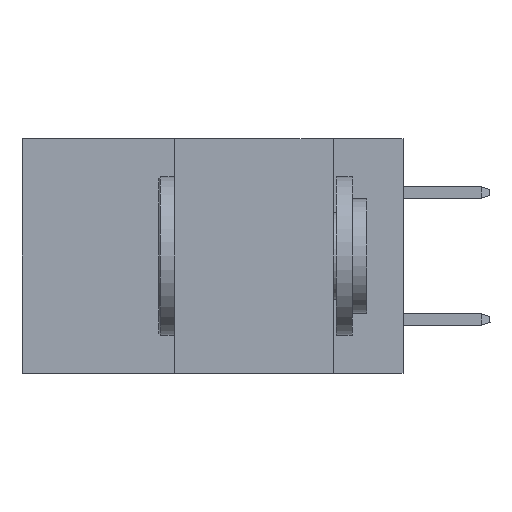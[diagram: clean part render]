
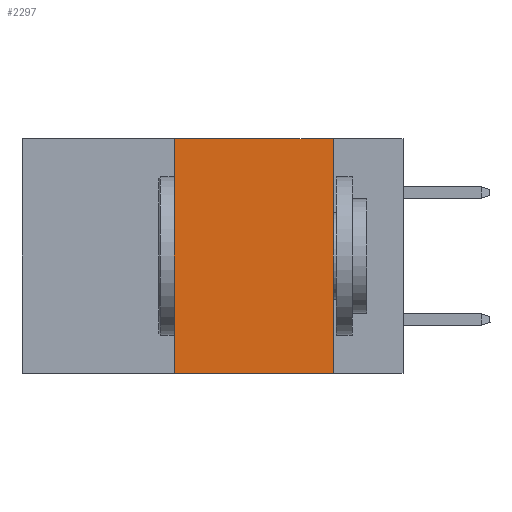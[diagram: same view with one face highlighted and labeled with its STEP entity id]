
A CAD part, left-side view. The second image highlights one B-rep face of the part: STEP entity #2297.
In plain terms, the highlighted planar face has unit normal (-1, 0, 0).
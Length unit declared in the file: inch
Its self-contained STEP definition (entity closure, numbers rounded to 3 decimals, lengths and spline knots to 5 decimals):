
#376 = VECTOR ( 'NONE', #2473, 39.37008 ) ;
#1329 = VECTOR ( 'NONE', #12461, 39.37008 ) ;
#2227 = EDGE_CURVE ( 'NONE', #12888, #9036, #9628, .T. ) ;
#2297 = ADVANCED_FACE ( 'NONE', ( #7451 ), #6273, .F. ) ;
#2473 = DIRECTION ( 'NONE',  ( 0., 0., -1. ) ) ;
#2727 = AXIS2_PLACEMENT_3D ( 'NONE', #7508, #8584, #14668 ) ;
#3053 = CARTESIAN_POINT ( 'NONE',  ( 0., 0.36, -0.37 ) ) ;
#3786 = CARTESIAN_POINT ( 'NONE',  ( 0., 0.11, 0. ) ) ;
#3841 = CARTESIAN_POINT ( 'NONE',  ( 0., 0.6, -0.37 ) ) ;
#4231 = EDGE_CURVE ( 'NONE', #9036, #7912, #9056, .T. ) ;
#4818 = CARTESIAN_POINT ( 'NONE',  ( 0., 0.36, 0. ) ) ;
#5990 = CARTESIAN_POINT ( 'NONE',  ( 0., 0.11, 0. ) ) ;
#6121 = VECTOR ( 'NONE', #11779, 39.37008 ) ;
#6273 = PLANE ( 'NONE',  #2727 ) ;
#7359 = ORIENTED_EDGE ( 'NONE', *, *, #11270, .F. ) ;
#7451 = FACE_OUTER_BOUND ( 'NONE', #11690, .T. ) ;
#7508 = CARTESIAN_POINT ( 'NONE',  ( 0., 0.6, 0. ) ) ;
#7912 = VERTEX_POINT ( 'NONE', #3786 ) ;
#8267 = EDGE_CURVE ( 'NONE', #12888, #11107, #13317, .T. ) ;
#8434 = DIRECTION ( 'NONE',  ( 0., -1., 0. ) ) ;
#8584 = DIRECTION ( 'NONE',  ( 1., 0., 0. ) ) ;
#8627 = ORIENTED_EDGE ( 'NONE', *, *, #4231, .F. ) ;
#8665 = CARTESIAN_POINT ( 'NONE',  ( 0., 0.11, -0.37 ) ) ;
#9036 = VERTEX_POINT ( 'NONE', #10922 ) ;
#9056 = LINE ( 'NONE', #11509, #1329 ) ;
#9628 = LINE ( 'NONE', #4818, #6121 ) ;
#10922 = CARTESIAN_POINT ( 'NONE',  ( 0., 0.36, 0. ) ) ;
#11107 = VERTEX_POINT ( 'NONE', #8665 ) ;
#11270 = EDGE_CURVE ( 'NONE', #7912, #11107, #11868, .T. ) ;
#11509 = CARTESIAN_POINT ( 'NONE',  ( 0., 0.6, 0. ) ) ;
#11690 = EDGE_LOOP ( 'NONE', ( #7359, #8627, #13456, #13478 ) ) ;
#11779 = DIRECTION ( 'NONE',  ( 0., 0., 1. ) ) ;
#11868 = LINE ( 'NONE', #5990, #376 ) ;
#12461 = DIRECTION ( 'NONE',  ( 0., -1., 0. ) ) ;
#12888 = VERTEX_POINT ( 'NONE', #3053 ) ;
#13317 = LINE ( 'NONE', #3841, #14350 ) ;
#13456 = ORIENTED_EDGE ( 'NONE', *, *, #2227, .F. ) ;
#13478 = ORIENTED_EDGE ( 'NONE', *, *, #8267, .T. ) ;
#14350 = VECTOR ( 'NONE', #8434, 39.37008 ) ;
#14668 = DIRECTION ( 'NONE',  ( 0., 0., -1. ) ) ;
